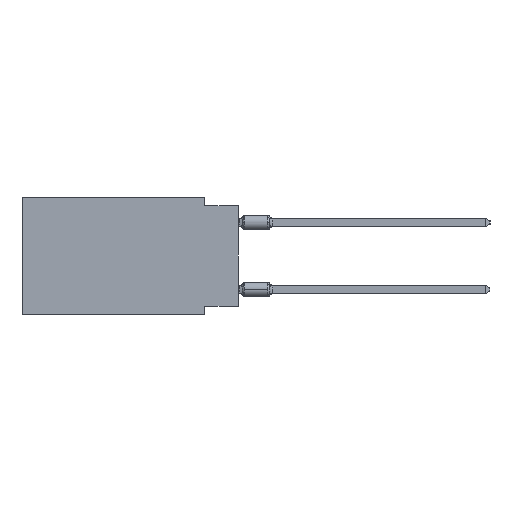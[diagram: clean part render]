
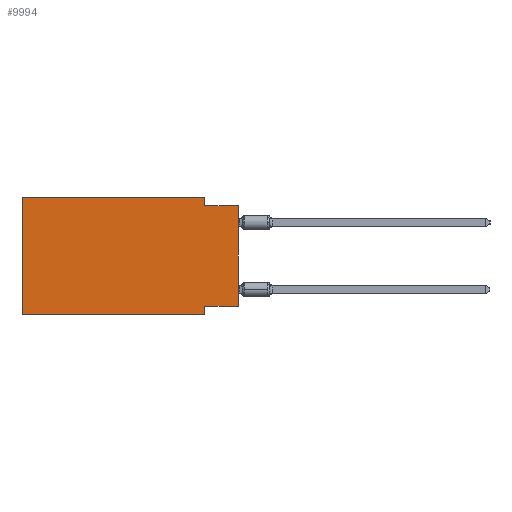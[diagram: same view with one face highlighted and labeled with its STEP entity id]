
A CAD part, left-side view. The second image highlights one B-rep face of the part: STEP entity #9994.
In plain terms, the highlighted planar face has unit normal (-1, 0, 0).
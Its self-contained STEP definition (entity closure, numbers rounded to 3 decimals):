
#2959 = ORIENTED_EDGE ( 'NONE', *, *, #37221, .F. ) ;
#3311 = CARTESIAN_POINT ( 'NONE',  ( 0., 0., -0.635 ) ) ;
#3447 = VECTOR ( 'NONE', #9543, 1000. ) ;
#4089 = DIRECTION ( 'NONE',  ( 0., 0., -1. ) ) ;
#5014 = DIRECTION ( 'NONE',  ( 0., 0., -1. ) ) ;
#5748 = CARTESIAN_POINT ( 'NONE',  ( 0., 2.54, -8.89 ) ) ;
#5978 = ORIENTED_EDGE ( 'NONE', *, *, #54951, .F. ) ;
#6669 = DIRECTION ( 'NONE',  ( 0., 1., 0. ) ) ;
#6923 = CARTESIAN_POINT ( 'NONE',  ( 0., 16.383, 0. ) ) ;
#7115 = VECTOR ( 'NONE', #34284, 1000. ) ;
#7500 = AXIS2_PLACEMENT_3D ( 'NONE', #27467, #41447, #60693 ) ;
#8763 = LINE ( 'NONE', #27714, #32478 ) ;
#9415 = ORIENTED_EDGE ( 'NONE', *, *, #26351, .F. ) ;
#9543 = DIRECTION ( 'NONE',  ( 0., 0., 1. ) ) ;
#9837 = VERTEX_POINT ( 'NONE', #5748 ) ;
#9994 = ADVANCED_FACE ( 'NONE', ( #37091 ), #50460, .F. ) ;
#10772 = CARTESIAN_POINT ( 'NONE',  ( 0., 0., 0. ) ) ;
#11064 = VERTEX_POINT ( 'NONE', #28478 ) ;
#12429 = DIRECTION ( 'NONE',  ( 0., -1., 0. ) ) ;
#12956 = VERTEX_POINT ( 'NONE', #56612 ) ;
#15301 = CARTESIAN_POINT ( 'NONE',  ( 0., 16.383, 0. ) ) ;
#15656 = EDGE_CURVE ( 'NONE', #12956, #35575, #56732, .T. ) ;
#15809 = EDGE_CURVE ( 'NONE', #35575, #47785, #49182, .T. ) ;
#17079 = ORIENTED_EDGE ( 'NONE', *, *, #15656, .F. ) ;
#17379 = CARTESIAN_POINT ( 'NONE',  ( 0., 0., -0.635 ) ) ;
#19682 = VECTOR ( 'NONE', #12429, 1000. ) ;
#21075 = VECTOR ( 'NONE', #60601, 1000. ) ;
#25867 = DIRECTION ( 'NONE',  ( 0., -1., 0. ) ) ;
#26351 = EDGE_CURVE ( 'NONE', #47229, #11064, #45190, .T. ) ;
#26841 = ORIENTED_EDGE ( 'NONE', *, *, #55842, .F. ) ;
#27467 = CARTESIAN_POINT ( 'NONE',  ( 0., 16.383, 0. ) ) ;
#27714 = CARTESIAN_POINT ( 'NONE',  ( 0., 2.54, 0. ) ) ;
#27972 = VECTOR ( 'NONE', #25867, 1000. ) ;
#28297 = LINE ( 'NONE', #60917, #21075 ) ;
#28478 = CARTESIAN_POINT ( 'NONE',  ( 0., 2.54, -8.255 ) ) ;
#29277 = EDGE_CURVE ( 'NONE', #12956, #9837, #28297, .T. ) ;
#31632 = EDGE_LOOP ( 'NONE', ( #55939, #5978, #2959, #41500, #17079, #34165, #26841, #9415 ) ) ;
#32478 = VECTOR ( 'NONE', #4089, 1000. ) ;
#34165 = ORIENTED_EDGE ( 'NONE', *, *, #29277, .T. ) ;
#34284 = DIRECTION ( 'NONE',  ( 0., 0., 1. ) ) ;
#35575 = VERTEX_POINT ( 'NONE', #50207 ) ;
#36948 = LINE ( 'NONE', #17379, #19682 ) ;
#37091 = FACE_OUTER_BOUND ( 'NONE', #31632, .T. ) ;
#37221 = EDGE_CURVE ( 'NONE', #47785, #59087, #8763, .T. ) ;
#41447 = DIRECTION ( 'NONE',  ( 1., 0., 0. ) ) ;
#41500 = ORIENTED_EDGE ( 'NONE', *, *, #15809, .F. ) ;
#42327 = LINE ( 'NONE', #42915, #48528 ) ;
#42915 = CARTESIAN_POINT ( 'NONE',  ( 0., 2.54, -8.89 ) ) ;
#43956 = EDGE_CURVE ( 'NONE', #47229, #51598, #48052, .T. ) ;
#45190 = LINE ( 'NONE', #59173, #49583 ) ;
#47229 = VERTEX_POINT ( 'NONE', #48192 ) ;
#47785 = VERTEX_POINT ( 'NONE', #49040 ) ;
#48052 = LINE ( 'NONE', #10772, #3447 ) ;
#48192 = CARTESIAN_POINT ( 'NONE',  ( 0., 0., -8.255 ) ) ;
#48528 = VECTOR ( 'NONE', #5014, 1000. ) ;
#49040 = CARTESIAN_POINT ( 'NONE',  ( 0., 2.54, 0. ) ) ;
#49182 = LINE ( 'NONE', #6923, #27972 ) ;
#49583 = VECTOR ( 'NONE', #6669, 1000. ) ;
#50207 = CARTESIAN_POINT ( 'NONE',  ( 0., 16.383, 0. ) ) ;
#50460 = PLANE ( 'NONE',  #7500 ) ;
#51598 = VERTEX_POINT ( 'NONE', #3311 ) ;
#54951 = EDGE_CURVE ( 'NONE', #59087, #51598, #36948, .T. ) ;
#55436 = CARTESIAN_POINT ( 'NONE',  ( 0., 2.54, -0.635 ) ) ;
#55842 = EDGE_CURVE ( 'NONE', #11064, #9837, #42327, .T. ) ;
#55939 = ORIENTED_EDGE ( 'NONE', *, *, #43956, .T. ) ;
#56612 = CARTESIAN_POINT ( 'NONE',  ( 0., 16.383, -8.89 ) ) ;
#56732 = LINE ( 'NONE', #15301, #7115 ) ;
#59087 = VERTEX_POINT ( 'NONE', #55436 ) ;
#59173 = CARTESIAN_POINT ( 'NONE',  ( 0., 0., -8.255 ) ) ;
#60601 = DIRECTION ( 'NONE',  ( 0., -1., 0. ) ) ;
#60693 = DIRECTION ( 'NONE',  ( 0., 0., -1. ) ) ;
#60917 = CARTESIAN_POINT ( 'NONE',  ( 0., 16.383, -8.89 ) ) ;
